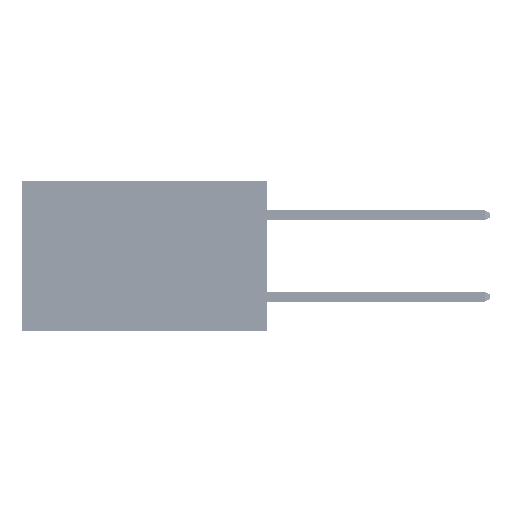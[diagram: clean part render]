
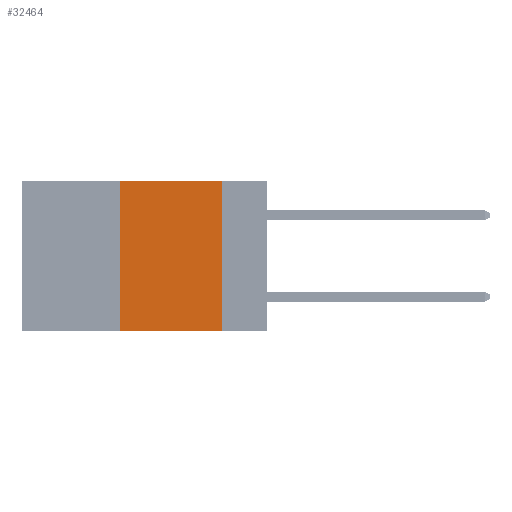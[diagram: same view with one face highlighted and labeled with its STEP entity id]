
A CAD part, left-side view. The second image highlights one B-rep face of the part: STEP entity #32464.
In plain terms, the highlighted planar face has unit normal (-1, 0, 0).
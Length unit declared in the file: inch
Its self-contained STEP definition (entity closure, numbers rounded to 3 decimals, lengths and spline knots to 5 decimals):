
#27 = LINE ( 'NONE', #47960, #8063 ) ;
#2291 = EDGE_CURVE ( 'NONE', #11671, #30907, #43456, .T. ) ;
#5919 = CARTESIAN_POINT ( 'NONE',  ( 0., 0.36, 0. ) ) ;
#6694 = DIRECTION ( 'NONE',  ( 0., 0., 1. ) ) ;
#8063 = VECTOR ( 'NONE', #28048, 39.37008 ) ;
#9329 = ORIENTED_EDGE ( 'NONE', *, *, #11819, .F. ) ;
#9551 = VERTEX_POINT ( 'NONE', #46861 ) ;
#11671 = VERTEX_POINT ( 'NONE', #5919 ) ;
#11819 = EDGE_CURVE ( 'NONE', #14990, #11671, #30285, .T. ) ;
#13956 = EDGE_LOOP ( 'NONE', ( #45940, #26272, #9329, #44330 ) ) ;
#14990 = VERTEX_POINT ( 'NONE', #22869 ) ;
#15297 = CARTESIAN_POINT ( 'NONE',  ( 0., 0.11, 0. ) ) ;
#15742 = DIRECTION ( 'NONE',  ( 0., 0., -1. ) ) ;
#17599 = CARTESIAN_POINT ( 'NONE',  ( 0., 0.11, 0. ) ) ;
#18440 = DIRECTION ( 'NONE',  ( 0., 0., -1. ) ) ;
#19656 = CARTESIAN_POINT ( 'NONE',  ( 0., 0.6, 0. ) ) ;
#19912 = FACE_OUTER_BOUND ( 'NONE', #13956, .T. ) ;
#22869 = CARTESIAN_POINT ( 'NONE',  ( 0., 0.36, -0.37 ) ) ;
#22901 = VECTOR ( 'NONE', #40035, 39.37008 ) ;
#24672 = EDGE_CURVE ( 'NONE', #14990, #9551, #27, .T. ) ;
#26272 = ORIENTED_EDGE ( 'NONE', *, *, #2291, .F. ) ;
#28048 = DIRECTION ( 'NONE',  ( 0., -1., 0. ) ) ;
#28253 = CARTESIAN_POINT ( 'NONE',  ( 0., 0.6, 0. ) ) ;
#30285 = LINE ( 'NONE', #50460, #42712 ) ;
#30907 = VERTEX_POINT ( 'NONE', #17599 ) ;
#31745 = AXIS2_PLACEMENT_3D ( 'NONE', #19656, #35677, #15742 ) ;
#32464 = ADVANCED_FACE ( 'NONE', ( #19912 ), #51168, .F. ) ;
#34978 = LINE ( 'NONE', #15297, #46549 ) ;
#35677 = DIRECTION ( 'NONE',  ( 1., 0., 0. ) ) ;
#40035 = DIRECTION ( 'NONE',  ( 0., -1., 0. ) ) ;
#41753 = EDGE_CURVE ( 'NONE', #30907, #9551, #34978, .T. ) ;
#42712 = VECTOR ( 'NONE', #6694, 39.37008 ) ;
#43456 = LINE ( 'NONE', #28253, #22901 ) ;
#44330 = ORIENTED_EDGE ( 'NONE', *, *, #24672, .T. ) ;
#45940 = ORIENTED_EDGE ( 'NONE', *, *, #41753, .F. ) ;
#46549 = VECTOR ( 'NONE', #18440, 39.37008 ) ;
#46861 = CARTESIAN_POINT ( 'NONE',  ( 0., 0.11, -0.37 ) ) ;
#47960 = CARTESIAN_POINT ( 'NONE',  ( 0., 0.6, -0.37 ) ) ;
#50460 = CARTESIAN_POINT ( 'NONE',  ( 0., 0.36, 0. ) ) ;
#51168 = PLANE ( 'NONE',  #31745 ) ;
